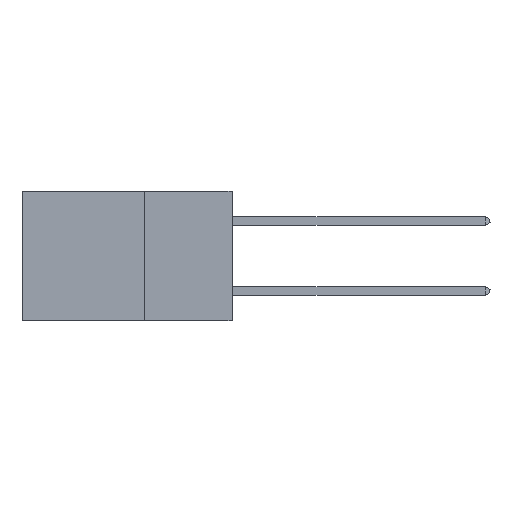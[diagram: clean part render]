
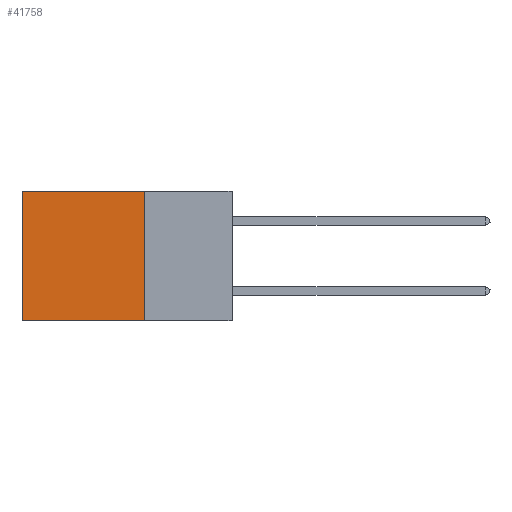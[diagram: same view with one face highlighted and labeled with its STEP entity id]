
A CAD part, left-side view. The second image highlights one B-rep face of the part: STEP entity #41758.
In plain terms, the highlighted planar face has unit normal (-1, 0, 0).
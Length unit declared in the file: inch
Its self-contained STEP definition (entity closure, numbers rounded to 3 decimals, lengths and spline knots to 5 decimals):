
#907 = EDGE_CURVE ( 'NONE', #18046, #30661, #26059, .T. ) ;
#3738 = AXIS2_PLACEMENT_3D ( 'NONE', #25675, #12154, #18398 ) ;
#4113 = CARTESIAN_POINT ( 'NONE',  ( 0.2875, 0.25, 0. ) ) ;
#4216 = FACE_OUTER_BOUND ( 'NONE', #9763, .T. ) ;
#5317 = EDGE_CURVE ( 'NONE', #30661, #16525, #17252, .T. ) ;
#6030 = VECTOR ( 'NONE', #40040, 39.37008 ) ;
#8774 = ORIENTED_EDGE ( 'NONE', *, *, #37310, .F. ) ;
#8807 = ORIENTED_EDGE ( 'NONE', *, *, #907, .T. ) ;
#9763 = EDGE_LOOP ( 'NONE', ( #31757, #28163, #8774, #8807 ) ) ;
#11781 = DIRECTION ( 'NONE',  ( 0., 0., -1. ) ) ;
#12154 = DIRECTION ( 'NONE',  ( 1., 0., 0. ) ) ;
#12212 = VECTOR ( 'NONE', #31316, 39.37008 ) ;
#13999 = CARTESIAN_POINT ( 'NONE',  ( 0.2875, 0.25, -0.37 ) ) ;
#14159 = CARTESIAN_POINT ( 'NONE',  ( 0.2875, 0.25, 0. ) ) ;
#14594 = VECTOR ( 'NONE', #28893, 39.37008 ) ;
#16525 = VERTEX_POINT ( 'NONE', #41626 ) ;
#17252 = LINE ( 'NONE', #38026, #14594 ) ;
#18046 = VERTEX_POINT ( 'NONE', #22351 ) ;
#18398 = DIRECTION ( 'NONE',  ( 0., 0., -1. ) ) ;
#18777 = LINE ( 'NONE', #30286, #6030 ) ;
#22351 = CARTESIAN_POINT ( 'NONE',  ( 0.2875, 0.25, 0. ) ) ;
#25675 = CARTESIAN_POINT ( 'NONE',  ( 0.2875, 0.25, 0. ) ) ;
#26059 = LINE ( 'NONE', #4113, #12212 ) ;
#28163 = ORIENTED_EDGE ( 'NONE', *, *, #34693, .F. ) ;
#28791 = PLANE ( 'NONE',  #3738 ) ;
#28893 = DIRECTION ( 'NONE',  ( 0., 0., -1. ) ) ;
#29291 = CARTESIAN_POINT ( 'NONE',  ( 0.2875, 0.6, 0. ) ) ;
#30286 = CARTESIAN_POINT ( 'NONE',  ( 0.2875, 0.25, -0.37 ) ) ;
#30661 = VERTEX_POINT ( 'NONE', #29291 ) ;
#31316 = DIRECTION ( 'NONE',  ( 0., 1., 0. ) ) ;
#31757 = ORIENTED_EDGE ( 'NONE', *, *, #5317, .T. ) ;
#33362 = VECTOR ( 'NONE', #11781, 39.37008 ) ;
#34693 = EDGE_CURVE ( 'NONE', #41680, #16525, #18777, .T. ) ;
#35481 = LINE ( 'NONE', #14159, #33362 ) ;
#37310 = EDGE_CURVE ( 'NONE', #18046, #41680, #35481, .T. ) ;
#38026 = CARTESIAN_POINT ( 'NONE',  ( 0.2875, 0.6, 0. ) ) ;
#40040 = DIRECTION ( 'NONE',  ( 0., 1., 0. ) ) ;
#41626 = CARTESIAN_POINT ( 'NONE',  ( 0.2875, 0.6, -0.37 ) ) ;
#41680 = VERTEX_POINT ( 'NONE', #13999 ) ;
#41758 = ADVANCED_FACE ( 'NONE', ( #4216 ), #28791, .F. ) ;
